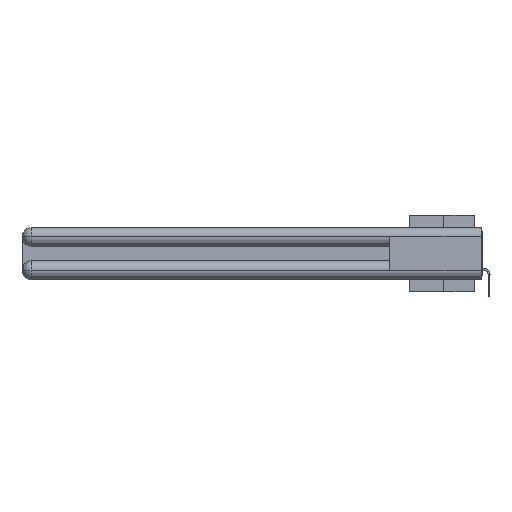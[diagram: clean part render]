
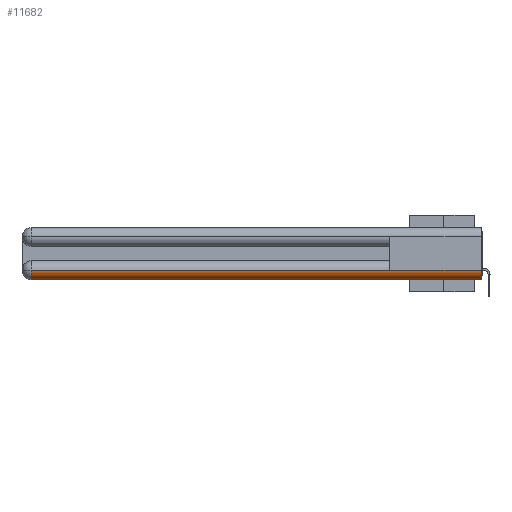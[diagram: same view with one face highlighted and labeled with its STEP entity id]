
A CAD part, left-side view. The second image highlights one B-rep face of the part: STEP entity #11682.
In plain terms, the highlighted cylindrical face has radius 1.562 mm (diameter 3.124 mm), a partial arc.
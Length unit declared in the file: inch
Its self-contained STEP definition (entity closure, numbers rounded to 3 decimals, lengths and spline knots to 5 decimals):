
#627 = EDGE_CURVE ( 'NONE', #5185, #14066, #27693, .T. ) ;
#1762 = CARTESIAN_POINT ( 'NONE',  ( 0.0615, 0., -0.2785 ) ) ;
#2724 = EDGE_CURVE ( 'NONE', #24487, #14066, #14245, .T. ) ;
#3894 = DIRECTION ( 'NONE',  ( 0., -1., 0. ) ) ;
#5185 = VERTEX_POINT ( 'NONE', #13132 ) ;
#5222 = CARTESIAN_POINT ( 'NONE',  ( 0., 0., -0.2785 ) ) ;
#5887 = DIRECTION ( 'NONE',  ( 0., 0., -1. ) ) ;
#7579 = DIRECTION ( 'NONE',  ( 0., 1., 0. ) ) ;
#8397 = CARTESIAN_POINT ( 'NONE',  ( 0.0615, 2.94, -0.34 ) ) ;
#8734 = FACE_OUTER_BOUND ( 'NONE', #12550, .T. ) ;
#9442 = ORIENTED_EDGE ( 'NONE', *, *, #26936, .F. ) ;
#9608 = CARTESIAN_POINT ( 'NONE',  ( 0.0615, 0., -0.34 ) ) ;
#11552 = EDGE_CURVE ( 'NONE', #14095, #24487, #12419, .T. ) ;
#11682 = ADVANCED_FACE ( 'NONE', ( #8734 ), #24648, .T. ) ;
#12130 = CARTESIAN_POINT ( 'NONE',  ( 0.0615, 0., -0.34 ) ) ;
#12419 = CIRCLE ( 'NONE', #27398, 0.0615 ) ;
#12550 = EDGE_LOOP ( 'NONE', ( #20789, #23523, #26952, #24676, #9442 ) ) ;
#13089 = CARTESIAN_POINT ( 'NONE',  ( 0., 0., -0.2785 ) ) ;
#13132 = CARTESIAN_POINT ( 'NONE',  ( 0., 2.94, -0.2785 ) ) ;
#14066 = VERTEX_POINT ( 'NONE', #8397 ) ;
#14095 = VERTEX_POINT ( 'NONE', #13089 ) ;
#14245 = LINE ( 'NONE', #12130, #24021 ) ;
#14647 = AXIS2_PLACEMENT_3D ( 'NONE', #19746, #29141, #26579 ) ;
#16801 = CARTESIAN_POINT ( 'NONE',  ( 0.0615, 0., -0.2785 ) ) ;
#19746 = CARTESIAN_POINT ( 'NONE',  ( 0.0615, 2.94, -0.2785 ) ) ;
#20789 = ORIENTED_EDGE ( 'NONE', *, *, #29578, .T. ) ;
#21219 = CARTESIAN_POINT ( 'NONE',  ( 0., 0., -0.2785 ) ) ;
#21424 = DIRECTION ( 'NONE',  ( 0., 1., 0. ) ) ;
#23488 = DIRECTION ( 'NONE',  ( 0., -1., 0. ) ) ;
#23523 = ORIENTED_EDGE ( 'NONE', *, *, #627, .T. ) ;
#23644 = LINE ( 'NONE', #21219, #26671 ) ;
#24021 = VECTOR ( 'NONE', #7579, 39.37008 ) ;
#24283 = LINE ( 'NONE', #5222, #27745 ) ;
#24487 = VERTEX_POINT ( 'NONE', #9608 ) ;
#24648 = CYLINDRICAL_SURFACE ( 'NONE', #27418, 0.0615 ) ;
#24676 = ORIENTED_EDGE ( 'NONE', *, *, #11552, .F. ) ;
#25890 = DIRECTION ( 'NONE',  ( 0., -1., 0. ) ) ;
#26579 = DIRECTION ( 'NONE',  ( 0., 0., 1. ) ) ;
#26671 = VECTOR ( 'NONE', #23488, 39.37008 ) ;
#26936 = EDGE_CURVE ( 'NONE', #27419, #14095, #23644, .T. ) ;
#26952 = ORIENTED_EDGE ( 'NONE', *, *, #2724, .F. ) ;
#27398 = AXIS2_PLACEMENT_3D ( 'NONE', #16801, #25890, #28166 ) ;
#27418 = AXIS2_PLACEMENT_3D ( 'NONE', #1762, #3894, #5887 ) ;
#27419 = VERTEX_POINT ( 'NONE', #28412 ) ;
#27693 = CIRCLE ( 'NONE', #14647, 0.0615 ) ;
#27745 = VECTOR ( 'NONE', #21424, 39.37008 ) ;
#28166 = DIRECTION ( 'NONE',  ( 1., 0., 0. ) ) ;
#28412 = CARTESIAN_POINT ( 'NONE',  ( 0., 0.6, -0.2785 ) ) ;
#29141 = DIRECTION ( 'NONE',  ( 0., -1., 0. ) ) ;
#29578 = EDGE_CURVE ( 'NONE', #27419, #5185, #24283, .T. ) ;
